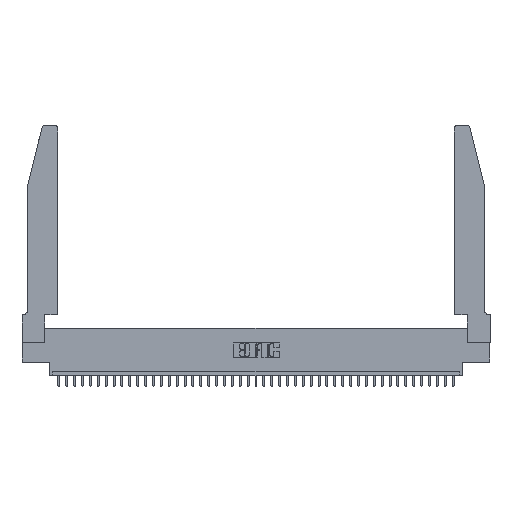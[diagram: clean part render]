
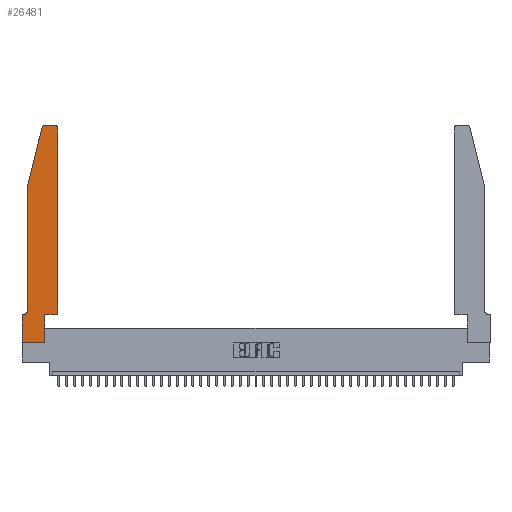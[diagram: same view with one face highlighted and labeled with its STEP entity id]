
A CAD part, top view. The second image highlights one B-rep face of the part: STEP entity #26481.
In plain terms, the highlighted planar face has unit normal (0, 0, 1).
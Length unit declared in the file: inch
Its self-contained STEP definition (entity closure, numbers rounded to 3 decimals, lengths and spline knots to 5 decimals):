
#1702 = DIRECTION ( 'NONE',  ( -1., 0., 0. ) ) ;
#1720 = DIRECTION ( 'NONE',  ( 1., 0., 0. ) ) ;
#2259 = EDGE_LOOP ( 'NONE', ( #23858, #28879, #33914, #35375, #14645, #6163, #39396, #41245, #31112, #28002, #29951, #13119 ) ) ;
#2554 = CARTESIAN_POINT ( 'NONE',  ( 0., 0., 0.37 ) ) ;
#3069 = FACE_OUTER_BOUND ( 'NONE', #2259, .T. ) ;
#3617 = DIRECTION ( 'NONE',  ( 1., 0., 0. ) ) ;
#3663 = EDGE_CURVE ( 'NONE', #8946, #30503, #10648, .T. ) ;
#4120 = VERTEX_POINT ( 'NONE', #24846 ) ;
#4594 = CARTESIAN_POINT ( 'NONE',  ( 0.2865, 0., 0.37 ) ) ;
#4700 = DIRECTION ( 'NONE',  ( 0., 0., 1. ) ) ;
#5130 = VECTOR ( 'NONE', #27827, 39.37008 ) ;
#5272 = VERTEX_POINT ( 'NONE', #6897 ) ;
#5374 = CARTESIAN_POINT ( 'NONE',  ( 0.2865, 0.35, 0.37 ) ) ;
#6119 = CARTESIAN_POINT ( 'NONE',  ( 0., 0., 0.37 ) ) ;
#6163 = ORIENTED_EDGE ( 'NONE', *, *, #27760, .T. ) ;
#6325 = EDGE_CURVE ( 'NONE', #5272, #10344, #32570, .T. ) ;
#6515 = CARTESIAN_POINT ( 'NONE',  ( 0.4205, 2.75, 0.37 ) ) ;
#6897 = CARTESIAN_POINT ( 'NONE',  ( 0.4505, 2.72, 0.37 ) ) ;
#7762 = CARTESIAN_POINT ( 'NONE',  ( 0.2605, 2.75, 0.37 ) ) ;
#7966 = VECTOR ( 'NONE', #36608, 39.37008 ) ;
#7981 = LINE ( 'NONE', #11245, #25225 ) ;
#8946 = VERTEX_POINT ( 'NONE', #28064 ) ;
#9186 = CARTESIAN_POINT ( 'NONE',  ( 0.0755, 2., 0.37 ) ) ;
#9863 = DIRECTION ( 'NONE',  ( 1., 0., 0. ) ) ;
#10344 = VERTEX_POINT ( 'NONE', #6515 ) ;
#10648 = LINE ( 'NONE', #2554, #36433 ) ;
#11245 = CARTESIAN_POINT ( 'NONE',  ( 0.0755, 2., 0.37 ) ) ;
#11940 = EDGE_CURVE ( 'NONE', #20778, #12287, #12775, .T. ) ;
#12287 = VERTEX_POINT ( 'NONE', #23676 ) ;
#12775 = CIRCLE ( 'NONE', #24755, 0.03 ) ;
#13119 = ORIENTED_EDGE ( 'NONE', *, *, #6325, .T. ) ;
#13725 = EDGE_CURVE ( 'NONE', #22837, #4120, #20152, .T. ) ;
#14160 = CARTESIAN_POINT ( 'NONE',  ( 0.4505, 0.35, 0.37 ) ) ;
#14645 = ORIENTED_EDGE ( 'NONE', *, *, #34080, .T. ) ;
#14733 = DIRECTION ( 'NONE',  ( 0., 0., 1. ) ) ;
#15217 = LINE ( 'NONE', #17810, #36913 ) ;
#15960 = CIRCLE ( 'NONE', #38229, 0.07 ) ;
#16961 = CARTESIAN_POINT ( 'NONE',  ( 0.284, 2.75, 0.37 ) ) ;
#17107 = DIRECTION ( 'NONE',  ( 0., 0., -1. ) ) ;
#17528 = DIRECTION ( 'NONE',  ( -1., 0., 0. ) ) ;
#17555 = CARTESIAN_POINT ( 'NONE',  ( 0.0755, 0.42, 0.37 ) ) ;
#17667 = EDGE_CURVE ( 'NONE', #4120, #5272, #36828, .T. ) ;
#17810 = CARTESIAN_POINT ( 'NONE',  ( 0.0755, 0.35, 0.37 ) ) ;
#20030 = VECTOR ( 'NONE', #35386, 39.37008 ) ;
#20152 = LINE ( 'NONE', #33034, #29249 ) ;
#20778 = VERTEX_POINT ( 'NONE', #16961 ) ;
#21459 = CARTESIAN_POINT ( 'NONE',  ( 0., 0.35, 0.37 ) ) ;
#22501 = EDGE_CURVE ( 'NONE', #24151, #27927, #7981, .T. ) ;
#22540 = DIRECTION ( 'NONE',  ( -0.239, -0.971, 0. ) ) ;
#22724 = EDGE_CURVE ( 'NONE', #10344, #20778, #27679, .T. ) ;
#22837 = VERTEX_POINT ( 'NONE', #5374 ) ;
#23009 = LINE ( 'NONE', #38631, #37276 ) ;
#23409 = CARTESIAN_POINT ( 'NONE',  ( 0.0055, 0.42, 0.37 ) ) ;
#23608 = EDGE_CURVE ( 'NONE', #28318, #8946, #31699, .T. ) ;
#23676 = CARTESIAN_POINT ( 'NONE',  ( 0.25487, 2.72718, 0.37 ) ) ;
#23858 = ORIENTED_EDGE ( 'NONE', *, *, #22724, .T. ) ;
#24151 = VERTEX_POINT ( 'NONE', #9186 ) ;
#24755 = AXIS2_PLACEMENT_3D ( 'NONE', #40954, #37950, #1720 ) ;
#24846 = CARTESIAN_POINT ( 'NONE',  ( 0.4505, 0.35, 0.37 ) ) ;
#24941 = AXIS2_PLACEMENT_3D ( 'NONE', #21459, #14733, #37361 ) ;
#25225 = VECTOR ( 'NONE', #33935, 39.37008 ) ;
#26440 = EDGE_CURVE ( 'NONE', #30503, #22837, #37029, .T. ) ;
#26481 = ADVANCED_FACE ( 'NONE', ( #3069 ), #37210, .T. ) ;
#27342 = DIRECTION ( 'NONE',  ( 1., 0., 0. ) ) ;
#27679 = LINE ( 'NONE', #7762, #33779 ) ;
#27760 = EDGE_CURVE ( 'NONE', #32659, #28318, #15217, .T. ) ;
#27827 = DIRECTION ( 'NONE',  ( 0., 1., 0. ) ) ;
#27927 = VERTEX_POINT ( 'NONE', #17555 ) ;
#28002 = ORIENTED_EDGE ( 'NONE', *, *, #13725, .T. ) ;
#28064 = CARTESIAN_POINT ( 'NONE',  ( 0., 0., 0.37 ) ) ;
#28318 = VERTEX_POINT ( 'NONE', #39228 ) ;
#28879 = ORIENTED_EDGE ( 'NONE', *, *, #11940, .T. ) ;
#29249 = VECTOR ( 'NONE', #3617, 39.37008 ) ;
#29951 = ORIENTED_EDGE ( 'NONE', *, *, #17667, .T. ) ;
#30503 = VERTEX_POINT ( 'NONE', #4594 ) ;
#31112 = ORIENTED_EDGE ( 'NONE', *, *, #26440, .T. ) ;
#31699 = LINE ( 'NONE', #6119, #20030 ) ;
#32386 = CARTESIAN_POINT ( 'NONE',  ( 0.0055, 0.35, 0.37 ) ) ;
#32570 = CIRCLE ( 'NONE', #39288, 0.03 ) ;
#32659 = VERTEX_POINT ( 'NONE', #32386 ) ;
#33011 = EDGE_CURVE ( 'NONE', #12287, #24151, #23009, .T. ) ;
#33034 = CARTESIAN_POINT ( 'NONE',  ( 0.4505, 0.35, 0.37 ) ) ;
#33779 = VECTOR ( 'NONE', #17528, 39.37008 ) ;
#33914 = ORIENTED_EDGE ( 'NONE', *, *, #33011, .T. ) ;
#33935 = DIRECTION ( 'NONE',  ( 0., -1., 0. ) ) ;
#34080 = EDGE_CURVE ( 'NONE', #27927, #32659, #15960, .T. ) ;
#35375 = ORIENTED_EDGE ( 'NONE', *, *, #22501, .T. ) ;
#35386 = DIRECTION ( 'NONE',  ( 0., -1., 0. ) ) ;
#36433 = VECTOR ( 'NONE', #9863, 39.37008 ) ;
#36608 = DIRECTION ( 'NONE',  ( 0., 1., 0. ) ) ;
#36828 = LINE ( 'NONE', #14160, #7966 ) ;
#36913 = VECTOR ( 'NONE', #1702, 39.37008 ) ;
#37020 = CARTESIAN_POINT ( 'NONE',  ( 0.4205, 2.72, 0.37 ) ) ;
#37029 = LINE ( 'NONE', #40810, #5130 ) ;
#37210 = PLANE ( 'NONE',  #24941 ) ;
#37276 = VECTOR ( 'NONE', #22540, 39.37008 ) ;
#37361 = DIRECTION ( 'NONE',  ( 1., 0., 0. ) ) ;
#37950 = DIRECTION ( 'NONE',  ( 0., 0., 1. ) ) ;
#38229 = AXIS2_PLACEMENT_3D ( 'NONE', #23409, #17107, #39792 ) ;
#38631 = CARTESIAN_POINT ( 'NONE',  ( 0.0755, 2., 0.37 ) ) ;
#39228 = CARTESIAN_POINT ( 'NONE',  ( 0., 0.35, 0.37 ) ) ;
#39288 = AXIS2_PLACEMENT_3D ( 'NONE', #37020, #4700, #27342 ) ;
#39396 = ORIENTED_EDGE ( 'NONE', *, *, #23608, .T. ) ;
#39792 = DIRECTION ( 'NONE',  ( -1., 0., 0. ) ) ;
#40810 = CARTESIAN_POINT ( 'NONE',  ( 0.2865, 0.35, 0.37 ) ) ;
#40954 = CARTESIAN_POINT ( 'NONE',  ( 0.284, 2.72, 0.37 ) ) ;
#41245 = ORIENTED_EDGE ( 'NONE', *, *, #3663, .T. ) ;
